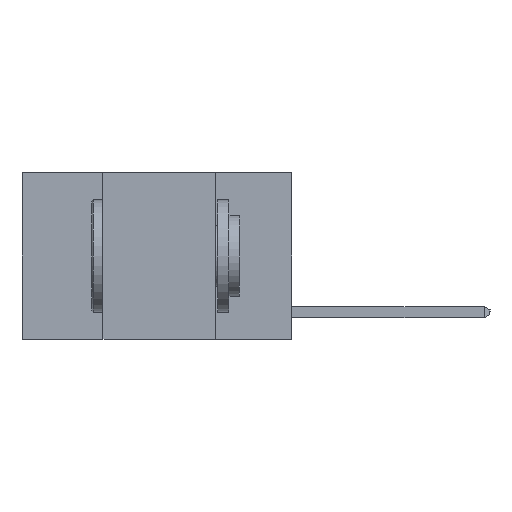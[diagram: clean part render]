
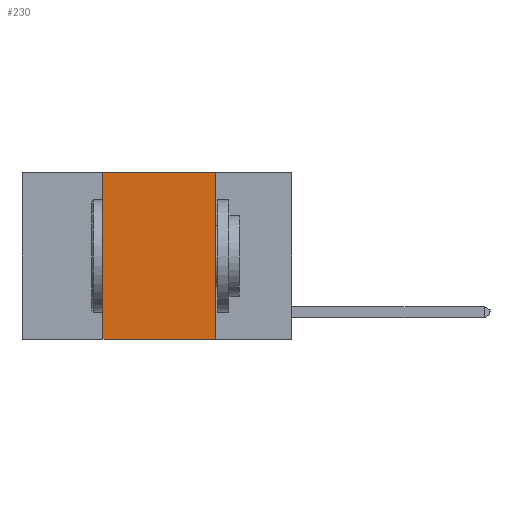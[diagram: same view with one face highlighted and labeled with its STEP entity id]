
A CAD part, left-side view. The second image highlights one B-rep face of the part: STEP entity #230.
In plain terms, the highlighted planar face has unit normal (-1, 0, 0).
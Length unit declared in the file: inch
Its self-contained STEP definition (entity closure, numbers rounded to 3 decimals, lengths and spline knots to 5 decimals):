
#230 = ADVANCED_FACE ( 'NONE', ( #6802 ), #12212, .F. ) ;
#1282 = VERTEX_POINT ( 'NONE', #10247 ) ;
#1386 = VECTOR ( 'NONE', #12913, 39.37008 ) ;
#1563 = VECTOR ( 'NONE', #13691, 39.37008 ) ;
#1618 = ORIENTED_EDGE ( 'NONE', *, *, #11580, .F. ) ;
#4107 = DIRECTION ( 'NONE',  ( 0., 0., 1. ) ) ;
#4969 = LINE ( 'NONE', #6021, #1563 ) ;
#5280 = CARTESIAN_POINT ( 'NONE',  ( 0., 0.6, -0.37 ) ) ;
#5289 = EDGE_LOOP ( 'NONE', ( #1618, #13211, #10620, #13624 ) ) ;
#6021 = CARTESIAN_POINT ( 'NONE',  ( 0., 0.17, 0. ) ) ;
#6780 = VERTEX_POINT ( 'NONE', #13425 ) ;
#6802 = FACE_OUTER_BOUND ( 'NONE', #5289, .T. ) ;
#7635 = VECTOR ( 'NONE', #16577, 39.37008 ) ;
#7735 = LINE ( 'NONE', #5280, #1386 ) ;
#7903 = CARTESIAN_POINT ( 'NONE',  ( 0., 0.17, 0. ) ) ;
#8275 = VERTEX_POINT ( 'NONE', #11258 ) ;
#9319 = AXIS2_PLACEMENT_3D ( 'NONE', #12594, #11392, #11332 ) ;
#10247 = CARTESIAN_POINT ( 'NONE',  ( 0., 0.17, -0.37 ) ) ;
#10329 = VECTOR ( 'NONE', #4107, 39.37008 ) ;
#10434 = CARTESIAN_POINT ( 'NONE',  ( 0., 0.42, 0. ) ) ;
#10620 = ORIENTED_EDGE ( 'NONE', *, *, #11850, .F. ) ;
#11101 = LINE ( 'NONE', #11426, #7635 ) ;
#11258 = CARTESIAN_POINT ( 'NONE',  ( 0., 0.42, 0. ) ) ;
#11332 = DIRECTION ( 'NONE',  ( 0., 0., -1. ) ) ;
#11392 = DIRECTION ( 'NONE',  ( 1., 0., 0. ) ) ;
#11426 = CARTESIAN_POINT ( 'NONE',  ( 0., 0.6, 0. ) ) ;
#11580 = EDGE_CURVE ( 'NONE', #16663, #1282, #4969, .T. ) ;
#11850 = EDGE_CURVE ( 'NONE', #6780, #8275, #13745, .T. ) ;
#12212 = PLANE ( 'NONE',  #9319 ) ;
#12594 = CARTESIAN_POINT ( 'NONE',  ( 0., 0.6, 0. ) ) ;
#12913 = DIRECTION ( 'NONE',  ( 0., -1., 0. ) ) ;
#13211 = ORIENTED_EDGE ( 'NONE', *, *, #16432, .F. ) ;
#13425 = CARTESIAN_POINT ( 'NONE',  ( 0., 0.42, -0.37 ) ) ;
#13442 = EDGE_CURVE ( 'NONE', #6780, #1282, #7735, .T. ) ;
#13624 = ORIENTED_EDGE ( 'NONE', *, *, #13442, .T. ) ;
#13691 = DIRECTION ( 'NONE',  ( 0., 0., -1. ) ) ;
#13745 = LINE ( 'NONE', #10434, #10329 ) ;
#16432 = EDGE_CURVE ( 'NONE', #8275, #16663, #11101, .T. ) ;
#16577 = DIRECTION ( 'NONE',  ( 0., -1., 0. ) ) ;
#16663 = VERTEX_POINT ( 'NONE', #7903 ) ;
